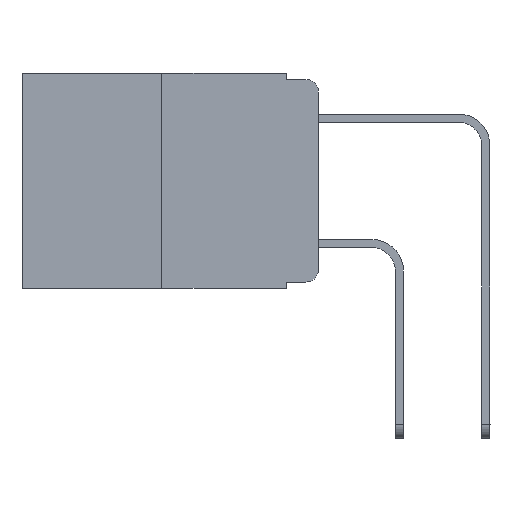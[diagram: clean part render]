
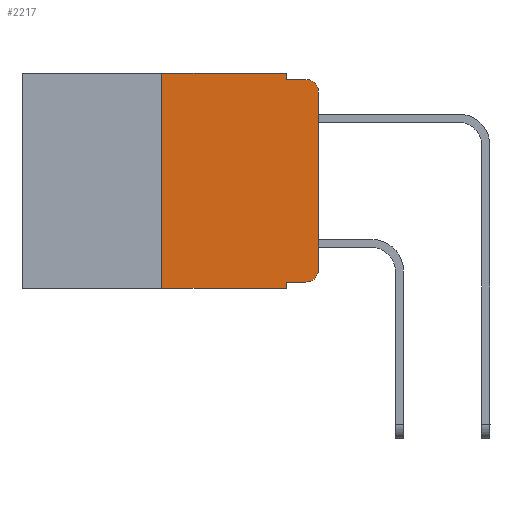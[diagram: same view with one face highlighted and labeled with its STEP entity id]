
A CAD part, left-side view. The second image highlights one B-rep face of the part: STEP entity #2217.
In plain terms, the highlighted planar face has unit normal (-1, 0, 0).
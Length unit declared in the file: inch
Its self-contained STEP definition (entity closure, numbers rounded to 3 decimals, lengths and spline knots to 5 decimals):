
#293 = CARTESIAN_POINT ( 'NONE',  ( 0., 0.02, -0.01 ) ) ;
#331 = ORIENTED_EDGE ( 'NONE', *, *, #5772, .T. ) ;
#729 = DIRECTION ( 'NONE',  ( 0., 0., -1. ) ) ;
#753 = DIRECTION ( 'NONE',  ( 0., 0., -1. ) ) ;
#1330 = DIRECTION ( 'NONE',  ( 0., -1., 0. ) ) ;
#1338 = CARTESIAN_POINT ( 'NONE',  ( 0., 0.473, 0. ) ) ;
#1360 = CARTESIAN_POINT ( 'NONE',  ( 0., 0.051, -0.01 ) ) ;
#1389 = EDGE_CURVE ( 'NONE', #12356, #13157, #6272, .T. ) ;
#1487 = CARTESIAN_POINT ( 'NONE',  ( 0., 0.051, -0.333 ) ) ;
#2070 = VECTOR ( 'NONE', #14178, 39.37008 ) ;
#2217 = ADVANCED_FACE ( 'NONE', ( #13997 ), #16735, .F. ) ;
#2271 = AXIS2_PLACEMENT_3D ( 'NONE', #15297, #7479, #11265 ) ;
#2365 = VERTEX_POINT ( 'NONE', #1360 ) ;
#2415 = CARTESIAN_POINT ( 'NONE',  ( 0., 0.051, -0.333 ) ) ;
#2507 = VERTEX_POINT ( 'NONE', #293 ) ;
#3003 = VECTOR ( 'NONE', #10687, 39.37008 ) ;
#3188 = VERTEX_POINT ( 'NONE', #9232 ) ;
#3385 = ORIENTED_EDGE ( 'NONE', *, *, #12582, .T. ) ;
#3515 = CARTESIAN_POINT ( 'NONE',  ( 0., 0., -0.03 ) ) ;
#3536 = CARTESIAN_POINT ( 'NONE',  ( 0., 0., -0.313 ) ) ;
#4317 = VECTOR ( 'NONE', #1330, 39.37008 ) ;
#4321 = EDGE_CURVE ( 'NONE', #13157, #2507, #6219, .T. ) ;
#4387 = LINE ( 'NONE', #1487, #12749 ) ;
#5162 = DIRECTION ( 'NONE',  ( 0., 0., 1. ) ) ;
#5297 = VERTEX_POINT ( 'NONE', #12091 ) ;
#5678 = LINE ( 'NONE', #17347, #3003 ) ;
#5700 = VECTOR ( 'NONE', #7831, 39.37008 ) ;
#5772 = EDGE_CURVE ( 'NONE', #11530, #5297, #6444, .T. ) ;
#5901 = CIRCLE ( 'NONE', #6778, 0.02 ) ;
#6107 = ORIENTED_EDGE ( 'NONE', *, *, #4321, .T. ) ;
#6219 = CIRCLE ( 'NONE', #2271, 0.02 ) ;
#6272 = LINE ( 'NONE', #11622, #5700 ) ;
#6312 = CARTESIAN_POINT ( 'NONE',  ( 0., 0.473, 0. ) ) ;
#6392 = CARTESIAN_POINT ( 'NONE',  ( 0., 0.25, -0.343 ) ) ;
#6444 = LINE ( 'NONE', #13284, #4317 ) ;
#6652 = VERTEX_POINT ( 'NONE', #10702 ) ;
#6778 = AXIS2_PLACEMENT_3D ( 'NONE', #7814, #10542, #7900 ) ;
#6928 = EDGE_CURVE ( 'NONE', #10428, #3188, #13203, .T. ) ;
#6975 = AXIS2_PLACEMENT_3D ( 'NONE', #6312, #9985, #753 ) ;
#6979 = ORIENTED_EDGE ( 'NONE', *, *, #16453, .F. ) ;
#7479 = DIRECTION ( 'NONE',  ( -1., 0., 0. ) ) ;
#7814 = CARTESIAN_POINT ( 'NONE',  ( 0., 0.02, -0.313 ) ) ;
#7831 = DIRECTION ( 'NONE',  ( 0., 0., 1. ) ) ;
#7900 = DIRECTION ( 'NONE',  ( 0., 0., -1. ) ) ;
#7954 = EDGE_CURVE ( 'NONE', #6652, #12356, #5901, .T. ) ;
#8716 = EDGE_CURVE ( 'NONE', #11510, #5297, #8918, .T. ) ;
#8918 = LINE ( 'NONE', #14250, #9542 ) ;
#9124 = LINE ( 'NONE', #15870, #15901 ) ;
#9133 = ORIENTED_EDGE ( 'NONE', *, *, #16235, .F. ) ;
#9232 = CARTESIAN_POINT ( 'NONE',  ( 0., 0.051, 0. ) ) ;
#9542 = VECTOR ( 'NONE', #10403, 39.37008 ) ;
#9696 = CARTESIAN_POINT ( 'NONE',  ( 0., 0.25, 0. ) ) ;
#9863 = ORIENTED_EDGE ( 'NONE', *, *, #8716, .F. ) ;
#9985 = DIRECTION ( 'NONE',  ( 1., 0., 0. ) ) ;
#10403 = DIRECTION ( 'NONE',  ( 0., 0., -1. ) ) ;
#10428 = VERTEX_POINT ( 'NONE', #9696 ) ;
#10542 = DIRECTION ( 'NONE',  ( -1., 0., 0. ) ) ;
#10687 = DIRECTION ( 'NONE',  ( 0., -1., 0. ) ) ;
#10702 = CARTESIAN_POINT ( 'NONE',  ( 0., 0.02, -0.333 ) ) ;
#11059 = DIRECTION ( 'NONE',  ( 0., -1., 0. ) ) ;
#11076 = ORIENTED_EDGE ( 'NONE', *, *, #7954, .T. ) ;
#11265 = DIRECTION ( 'NONE',  ( 0., 0., -1. ) ) ;
#11510 = VERTEX_POINT ( 'NONE', #2415 ) ;
#11530 = VERTEX_POINT ( 'NONE', #6392 ) ;
#11622 = CARTESIAN_POINT ( 'NONE',  ( 0., 0., 0. ) ) ;
#12091 = CARTESIAN_POINT ( 'NONE',  ( 0., 0.051, -0.343 ) ) ;
#12222 = ORIENTED_EDGE ( 'NONE', *, *, #15187, .F. ) ;
#12356 = VERTEX_POINT ( 'NONE', #3536 ) ;
#12582 = EDGE_CURVE ( 'NONE', #11510, #6652, #4387, .T. ) ;
#12749 = VECTOR ( 'NONE', #11059, 39.37008 ) ;
#13157 = VERTEX_POINT ( 'NONE', #3515 ) ;
#13203 = LINE ( 'NONE', #1338, #2070 ) ;
#13237 = ORIENTED_EDGE ( 'NONE', *, *, #1389, .T. ) ;
#13284 = CARTESIAN_POINT ( 'NONE',  ( 0., 0.473, -0.343 ) ) ;
#13978 = LINE ( 'NONE', #15316, #17253 ) ;
#13997 = FACE_OUTER_BOUND ( 'NONE', #16559, .T. ) ;
#14178 = DIRECTION ( 'NONE',  ( 0., -1., 0. ) ) ;
#14250 = CARTESIAN_POINT ( 'NONE',  ( 0., 0.051, 0. ) ) ;
#15187 = EDGE_CURVE ( 'NONE', #3188, #2365, #13978, .T. ) ;
#15297 = CARTESIAN_POINT ( 'NONE',  ( 0., 0.02, -0.03 ) ) ;
#15316 = CARTESIAN_POINT ( 'NONE',  ( 0., 0.051, 0. ) ) ;
#15870 = CARTESIAN_POINT ( 'NONE',  ( 0., 0.25, 0. ) ) ;
#15901 = VECTOR ( 'NONE', #5162, 39.37008 ) ;
#16235 = EDGE_CURVE ( 'NONE', #11530, #10428, #9124, .T. ) ;
#16453 = EDGE_CURVE ( 'NONE', #2365, #2507, #5678, .T. ) ;
#16559 = EDGE_LOOP ( 'NONE', ( #13237, #6107, #6979, #12222, #16926, #9133, #331, #9863, #3385, #11076 ) ) ;
#16735 = PLANE ( 'NONE',  #6975 ) ;
#16926 = ORIENTED_EDGE ( 'NONE', *, *, #6928, .F. ) ;
#17253 = VECTOR ( 'NONE', #729, 39.37008 ) ;
#17347 = CARTESIAN_POINT ( 'NONE',  ( 0., 0.051, -0.01 ) ) ;
